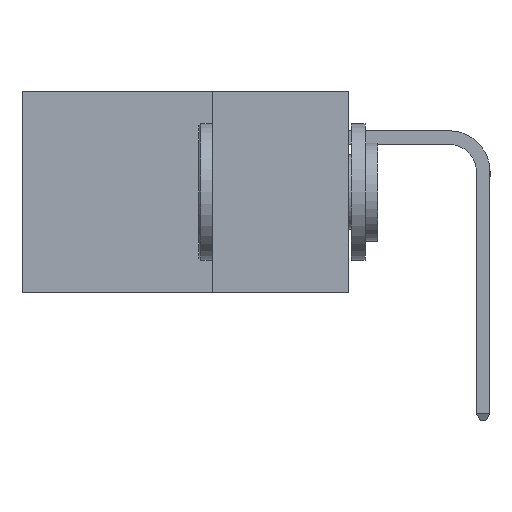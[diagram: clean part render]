
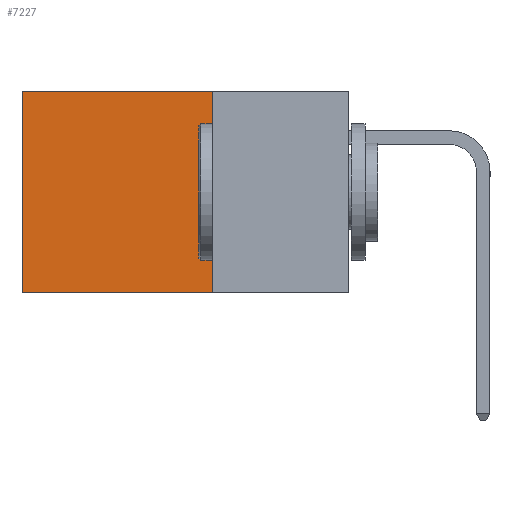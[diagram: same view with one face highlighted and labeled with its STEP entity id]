
A CAD part, left-side view. The second image highlights one B-rep face of the part: STEP entity #7227.
In plain terms, the highlighted planar face has unit normal (-1, 0, 0).
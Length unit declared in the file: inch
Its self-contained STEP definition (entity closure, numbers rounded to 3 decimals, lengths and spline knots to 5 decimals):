
#103 = CARTESIAN_POINT ( 'NONE',  ( 0.2875, 0.25, -0.37 ) ) ;
#426 = AXIS2_PLACEMENT_3D ( 'NONE', #2843, #2894, #9649 ) ;
#503 = ORIENTED_EDGE ( 'NONE', *, *, #7575, .T. ) ;
#985 = EDGE_CURVE ( 'NONE', #1754, #4339, #5639, .T. ) ;
#1754 = VERTEX_POINT ( 'NONE', #7492 ) ;
#2669 = VECTOR ( 'NONE', #3694, 39.37008 ) ;
#2843 = CARTESIAN_POINT ( 'NONE',  ( 0.2875, 0.25, 0. ) ) ;
#2894 = DIRECTION ( 'NONE',  ( 1., 0., 0. ) ) ;
#3157 = CARTESIAN_POINT ( 'NONE',  ( 0.2875, 0.6, -0.37 ) ) ;
#3212 = EDGE_CURVE ( 'NONE', #1754, #9899, #9823, .T. ) ;
#3260 = LINE ( 'NONE', #6356, #9738 ) ;
#3694 = DIRECTION ( 'NONE',  ( 0., 1., 0. ) ) ;
#3705 = LINE ( 'NONE', #103, #6656 ) ;
#3956 = CARTESIAN_POINT ( 'NONE',  ( 0.2875, 0.25, 0. ) ) ;
#4339 = VERTEX_POINT ( 'NONE', #7280 ) ;
#4560 = EDGE_LOOP ( 'NONE', ( #503, #12370, #8750, #9065 ) ) ;
#5639 = LINE ( 'NONE', #3956, #2669 ) ;
#6089 = VERTEX_POINT ( 'NONE', #3157 ) ;
#6356 = CARTESIAN_POINT ( 'NONE',  ( 0.2875, 0.6, 0. ) ) ;
#6656 = VECTOR ( 'NONE', #9980, 39.37008 ) ;
#7227 = ADVANCED_FACE ( 'NONE', ( #11039 ), #12369, .F. ) ;
#7280 = CARTESIAN_POINT ( 'NONE',  ( 0.2875, 0.6, 0. ) ) ;
#7379 = VECTOR ( 'NONE', #11203, 39.37008 ) ;
#7492 = CARTESIAN_POINT ( 'NONE',  ( 0.2875, 0.25, 0. ) ) ;
#7575 = EDGE_CURVE ( 'NONE', #4339, #6089, #3260, .T. ) ;
#8711 = EDGE_CURVE ( 'NONE', #9899, #6089, #3705, .T. ) ;
#8750 = ORIENTED_EDGE ( 'NONE', *, *, #3212, .F. ) ;
#9065 = ORIENTED_EDGE ( 'NONE', *, *, #985, .T. ) ;
#9649 = DIRECTION ( 'NONE',  ( 0., 0., -1. ) ) ;
#9738 = VECTOR ( 'NONE', #11008, 39.37008 ) ;
#9823 = LINE ( 'NONE', #11306, #7379 ) ;
#9899 = VERTEX_POINT ( 'NONE', #11226 ) ;
#9980 = DIRECTION ( 'NONE',  ( 0., 1., 0. ) ) ;
#11008 = DIRECTION ( 'NONE',  ( 0., 0., -1. ) ) ;
#11039 = FACE_OUTER_BOUND ( 'NONE', #4560, .T. ) ;
#11203 = DIRECTION ( 'NONE',  ( 0., 0., -1. ) ) ;
#11226 = CARTESIAN_POINT ( 'NONE',  ( 0.2875, 0.25, -0.37 ) ) ;
#11306 = CARTESIAN_POINT ( 'NONE',  ( 0.2875, 0.25, 0. ) ) ;
#12369 = PLANE ( 'NONE',  #426 ) ;
#12370 = ORIENTED_EDGE ( 'NONE', *, *, #8711, .F. ) ;
